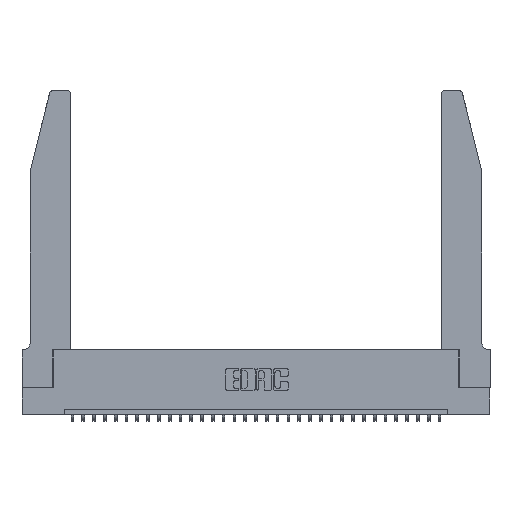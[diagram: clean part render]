
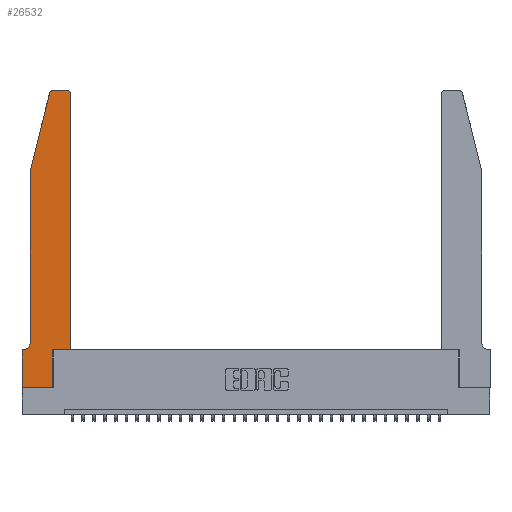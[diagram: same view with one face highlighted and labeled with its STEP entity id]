
A CAD part, top view. The second image highlights one B-rep face of the part: STEP entity #26532.
In plain terms, the highlighted planar face has unit normal (0, 0, 1).
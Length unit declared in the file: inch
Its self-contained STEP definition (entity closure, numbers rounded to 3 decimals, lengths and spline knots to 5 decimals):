
#260 = DIRECTION ( 'NONE',  ( -1., 0., 0. ) ) ;
#1498 = CARTESIAN_POINT ( 'NONE',  ( 0.0755, 2., 0.37 ) ) ;
#1567 = CARTESIAN_POINT ( 'NONE',  ( 0.2865, 0.35, 0.37 ) ) ;
#1695 = DIRECTION ( 'NONE',  ( 1., 0., 0. ) ) ;
#1721 = ORIENTED_EDGE ( 'NONE', *, *, #15696, .T. ) ;
#1987 = LINE ( 'NONE', #18014, #26056 ) ;
#2311 = VECTOR ( 'NONE', #19006, 39.37008 ) ;
#3295 = CARTESIAN_POINT ( 'NONE',  ( 0.0755, 2., 0.37 ) ) ;
#3378 = EDGE_CURVE ( 'NONE', #8669, #23142, #25560, .T. ) ;
#3793 = EDGE_LOOP ( 'NONE', ( #22648, #28332, #29431, #24620, #7493, #4022, #1721, #17986, #9362, #15269, #13613, #24801 ) ) ;
#3803 = CIRCLE ( 'NONE', #30140, 0.07 ) ;
#4022 = ORIENTED_EDGE ( 'NONE', *, *, #7449, .T. ) ;
#5008 = CARTESIAN_POINT ( 'NONE',  ( 0.4505, 0.35, 0.37 ) ) ;
#5241 = DIRECTION ( 'NONE',  ( 0., -1., 0. ) ) ;
#5442 = LINE ( 'NONE', #1498, #2311 ) ;
#5505 = CARTESIAN_POINT ( 'NONE',  ( 0., 0., 0.37 ) ) ;
#5597 = EDGE_CURVE ( 'NONE', #5711, #14509, #22726, .T. ) ;
#5659 = CARTESIAN_POINT ( 'NONE',  ( 0.25487, 2.72718, 0.37 ) ) ;
#5664 = DIRECTION ( 'NONE',  ( -1., 0., 0. ) ) ;
#5711 = VERTEX_POINT ( 'NONE', #5008 ) ;
#5902 = CARTESIAN_POINT ( 'NONE',  ( 0.4505, 2.72, 0.37 ) ) ;
#5916 = DIRECTION ( 'NONE',  ( 0., 0., 1. ) ) ;
#5982 = CARTESIAN_POINT ( 'NONE',  ( 0.2865, 0.35, 0.37 ) ) ;
#7449 = EDGE_CURVE ( 'NONE', #21911, #27812, #25021, .T. ) ;
#7493 = ORIENTED_EDGE ( 'NONE', *, *, #11662, .T. ) ;
#8503 = VECTOR ( 'NONE', #18862, 39.37008 ) ;
#8551 = EDGE_CURVE ( 'NONE', #9733, #8669, #24212, .T. ) ;
#8669 = VERTEX_POINT ( 'NONE', #30432 ) ;
#8712 = LINE ( 'NONE', #20109, #24228 ) ;
#9101 = AXIS2_PLACEMENT_3D ( 'NONE', #15879, #30688, #31013 ) ;
#9247 = FACE_OUTER_BOUND ( 'NONE', #3793, .T. ) ;
#9362 = ORIENTED_EDGE ( 'NONE', *, *, #3378, .T. ) ;
#9733 = VERTEX_POINT ( 'NONE', #20921 ) ;
#10010 = DIRECTION ( 'NONE',  ( -1., 0., 0. ) ) ;
#10091 = AXIS2_PLACEMENT_3D ( 'NONE', #14100, #16491, #1695 ) ;
#10442 = CIRCLE ( 'NONE', #10091, 0.03 ) ;
#11008 = DIRECTION ( 'NONE',  ( 1., 0., 0. ) ) ;
#11637 = CARTESIAN_POINT ( 'NONE',  ( 0.0055, 0.35, 0.37 ) ) ;
#11662 = EDGE_CURVE ( 'NONE', #13266, #21911, #3803, .T. ) ;
#12725 = CARTESIAN_POINT ( 'NONE',  ( 0.0755, 0.35, 0.37 ) ) ;
#13266 = VERTEX_POINT ( 'NONE', #25673 ) ;
#13282 = VECTOR ( 'NONE', #20189, 39.37008 ) ;
#13613 = ORIENTED_EDGE ( 'NONE', *, *, #5597, .T. ) ;
#14069 = VERTEX_POINT ( 'NONE', #19117 ) ;
#14100 = CARTESIAN_POINT ( 'NONE',  ( 0.284, 2.72, 0.37 ) ) ;
#14232 = AXIS2_PLACEMENT_3D ( 'NONE', #23042, #5916, #11008 ) ;
#14509 = VERTEX_POINT ( 'NONE', #5902 ) ;
#15238 = LINE ( 'NONE', #3295, #13282 ) ;
#15269 = ORIENTED_EDGE ( 'NONE', *, *, #22010, .T. ) ;
#15696 = EDGE_CURVE ( 'NONE', #27812, #9733, #8712, .T. ) ;
#15879 = CARTESIAN_POINT ( 'NONE',  ( 0.4205, 2.72, 0.37 ) ) ;
#16491 = DIRECTION ( 'NONE',  ( 0., 0., 1. ) ) ;
#16836 = EDGE_CURVE ( 'NONE', #30708, #13266, #15238, .T. ) ;
#17591 = CARTESIAN_POINT ( 'NONE',  ( 0., 0.35, 0.37 ) ) ;
#17744 = VERTEX_POINT ( 'NONE', #5659 ) ;
#17889 = EDGE_CURVE ( 'NONE', #17744, #30708, #5442, .T. ) ;
#17986 = ORIENTED_EDGE ( 'NONE', *, *, #8551, .T. ) ;
#18014 = CARTESIAN_POINT ( 'NONE',  ( 0.2605, 2.75, 0.37 ) ) ;
#18388 = PLANE ( 'NONE',  #14232 ) ;
#18835 = VECTOR ( 'NONE', #23864, 39.37008 ) ;
#18862 = DIRECTION ( 'NONE',  ( 0., 1., 0. ) ) ;
#19006 = DIRECTION ( 'NONE',  ( -0.239, -0.971, 0. ) ) ;
#19117 = CARTESIAN_POINT ( 'NONE',  ( 0.284, 2.75, 0.37 ) ) ;
#19210 = LINE ( 'NONE', #20369, #18835 ) ;
#20109 = CARTESIAN_POINT ( 'NONE',  ( 0., 0., 0.37 ) ) ;
#20189 = DIRECTION ( 'NONE',  ( 0., -1., 0. ) ) ;
#20369 = CARTESIAN_POINT ( 'NONE',  ( 0.4505, 0.35, 0.37 ) ) ;
#20708 = VECTOR ( 'NONE', #22858, 39.37008 ) ;
#20921 = CARTESIAN_POINT ( 'NONE',  ( 0., 0., 0.37 ) ) ;
#21911 = VERTEX_POINT ( 'NONE', #11637 ) ;
#22010 = EDGE_CURVE ( 'NONE', #23142, #5711, #19210, .T. ) ;
#22522 = DIRECTION ( 'NONE',  ( 0., 0., -1. ) ) ;
#22648 = ORIENTED_EDGE ( 'NONE', *, *, #29926, .T. ) ;
#22726 = LINE ( 'NONE', #24182, #31657 ) ;
#22858 = DIRECTION ( 'NONE',  ( 1., 0., 0. ) ) ;
#23042 = CARTESIAN_POINT ( 'NONE',  ( 0., 0.35, 0.37 ) ) ;
#23142 = VERTEX_POINT ( 'NONE', #5982 ) ;
#23518 = CARTESIAN_POINT ( 'NONE',  ( 0.0755, 2., 0.37 ) ) ;
#23864 = DIRECTION ( 'NONE',  ( 1., 0., 0. ) ) ;
#24182 = CARTESIAN_POINT ( 'NONE',  ( 0.4505, 0.35, 0.37 ) ) ;
#24201 = CARTESIAN_POINT ( 'NONE',  ( 0.4205, 2.75, 0.37 ) ) ;
#24212 = LINE ( 'NONE', #5505, #20708 ) ;
#24228 = VECTOR ( 'NONE', #5241, 39.37008 ) ;
#24271 = VECTOR ( 'NONE', #10010, 39.37008 ) ;
#24620 = ORIENTED_EDGE ( 'NONE', *, *, #16836, .T. ) ;
#24801 = ORIENTED_EDGE ( 'NONE', *, *, #29979, .T. ) ;
#25021 = LINE ( 'NONE', #12725, #24271 ) ;
#25560 = LINE ( 'NONE', #1567, #8503 ) ;
#25673 = CARTESIAN_POINT ( 'NONE',  ( 0.0755, 0.42, 0.37 ) ) ;
#25914 = VERTEX_POINT ( 'NONE', #24201 ) ;
#26056 = VECTOR ( 'NONE', #5664, 39.37008 ) ;
#26532 = ADVANCED_FACE ( 'NONE', ( #9247 ), #18388, .T. ) ;
#26826 = CIRCLE ( 'NONE', #9101, 0.03 ) ;
#27409 = CARTESIAN_POINT ( 'NONE',  ( 0.0055, 0.42, 0.37 ) ) ;
#27812 = VERTEX_POINT ( 'NONE', #17591 ) ;
#28332 = ORIENTED_EDGE ( 'NONE', *, *, #30874, .T. ) ;
#29431 = ORIENTED_EDGE ( 'NONE', *, *, #17889, .T. ) ;
#29926 = EDGE_CURVE ( 'NONE', #25914, #14069, #1987, .T. ) ;
#29979 = EDGE_CURVE ( 'NONE', #14509, #25914, #26826, .T. ) ;
#30140 = AXIS2_PLACEMENT_3D ( 'NONE', #27409, #22522, #260 ) ;
#30432 = CARTESIAN_POINT ( 'NONE',  ( 0.2865, 0., 0.37 ) ) ;
#30688 = DIRECTION ( 'NONE',  ( 0., 0., 1. ) ) ;
#30708 = VERTEX_POINT ( 'NONE', #23518 ) ;
#30874 = EDGE_CURVE ( 'NONE', #14069, #17744, #10442, .T. ) ;
#31013 = DIRECTION ( 'NONE',  ( 1., 0., 0. ) ) ;
#31419 = DIRECTION ( 'NONE',  ( 0., 1., 0. ) ) ;
#31657 = VECTOR ( 'NONE', #31419, 39.37008 ) ;
